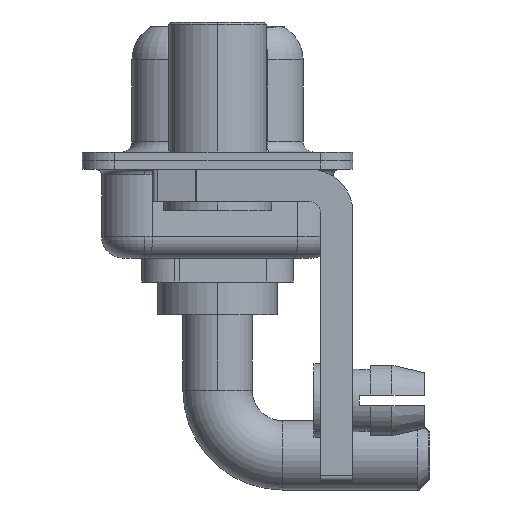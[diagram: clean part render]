
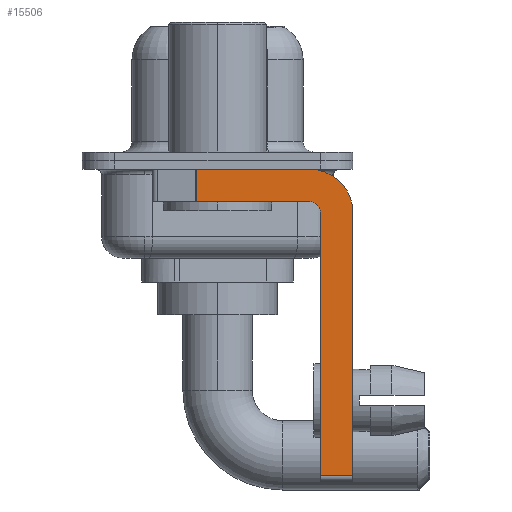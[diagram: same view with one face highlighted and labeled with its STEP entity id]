
A CAD part, left-side view. The second image highlights one B-rep face of the part: STEP entity #15506.
In plain terms, the highlighted planar face has unit normal (-1, 0, 0).
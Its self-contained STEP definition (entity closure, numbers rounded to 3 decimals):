
#155 = CARTESIAN_POINT ( 'NONE',  ( -2.9, -4.75, -2.4 ) ) ;
#188 = EDGE_CURVE ( 'NONE', #5756, #12203, #13516, .T. ) ;
#191 = PLANE ( 'NONE',  #10311 ) ;
#563 = VECTOR ( 'NONE', #5651, 1000. ) ;
#1056 = VERTEX_POINT ( 'NONE', #3633 ) ;
#1545 = ORIENTED_EDGE ( 'NONE', *, *, #10931, .F. ) ;
#1549 = CARTESIAN_POINT ( 'NONE',  ( -2.9, 0.978, -1.9 ) ) ;
#1575 = CARTESIAN_POINT ( 'NONE',  ( -2.9, -4.25, -14.55 ) ) ;
#2806 = CIRCLE ( 'NONE', #4302, 2. ) ;
#2824 = EDGE_CURVE ( 'NONE', #4322, #5120, #13715, .T. ) ;
#3224 = ORIENTED_EDGE ( 'NONE', *, *, #15464, .F. ) ;
#3633 = CARTESIAN_POINT ( 'NONE',  ( -2.9, -4.25, -0.4 ) ) ;
#4158 = DIRECTION ( 'NONE',  ( 1., 0., 0. ) ) ;
#4302 = AXIS2_PLACEMENT_3D ( 'NONE', #16575, #4158, #4515 ) ;
#4322 = VERTEX_POINT ( 'NONE', #9984 ) ;
#4487 = DIRECTION ( 'NONE',  ( -1., 0., 0. ) ) ;
#4515 = DIRECTION ( 'NONE',  ( 0., 0., -1. ) ) ;
#4554 = EDGE_CURVE ( 'NONE', #4322, #5756, #16165, .T. ) ;
#5057 = VECTOR ( 'NONE', #6839, 1000. ) ;
#5118 = CARTESIAN_POINT ( 'NONE',  ( -2.9, 3., -0.4 ) ) ;
#5120 = VERTEX_POINT ( 'NONE', #5518 ) ;
#5518 = CARTESIAN_POINT ( 'NONE',  ( -2.9, -6.25, -14.55 ) ) ;
#5614 = FACE_OUTER_BOUND ( 'NONE', #17122, .T. ) ;
#5629 = CARTESIAN_POINT ( 'NONE',  ( -2.9, -4.75, -14.8 ) ) ;
#5651 = DIRECTION ( 'NONE',  ( 0., -1., 0. ) ) ;
#5690 = AXIS2_PLACEMENT_3D ( 'NONE', #16894, #4487, #11078 ) ;
#5756 = VERTEX_POINT ( 'NONE', #155 ) ;
#5788 = ORIENTED_EDGE ( 'NONE', *, *, #4554, .F. ) ;
#5887 = LINE ( 'NONE', #1549, #11136 ) ;
#6839 = DIRECTION ( 'NONE',  ( 0., 0., -1. ) ) ;
#7161 = DIRECTION ( 'NONE',  ( 1., 0., 0. ) ) ;
#7304 = EDGE_CURVE ( 'NONE', #14701, #5120, #10545, .T. ) ;
#8168 = DIRECTION ( 'NONE',  ( 0., 0., 1. ) ) ;
#8398 = CARTESIAN_POINT ( 'NONE',  ( -2.9, -4.25, -1.9 ) ) ;
#8458 = CARTESIAN_POINT ( 'NONE',  ( -2.9, -6.25, -2.4 ) ) ;
#8648 = VERTEX_POINT ( 'NONE', #11760 ) ;
#8921 = ORIENTED_EDGE ( 'NONE', *, *, #188, .F. ) ;
#9684 = LINE ( 'NONE', #12331, #11187 ) ;
#9984 = CARTESIAN_POINT ( 'NONE',  ( -2.9, -4.75, -14.55 ) ) ;
#10311 = AXIS2_PLACEMENT_3D ( 'NONE', #12509, #7161, #17876 ) ;
#10453 = EDGE_CURVE ( 'NONE', #1056, #14701, #2806, .T. ) ;
#10545 = LINE ( 'NONE', #14737, #5057 ) ;
#10931 = EDGE_CURVE ( 'NONE', #14274, #1056, #14447, .T. ) ;
#11032 = VECTOR ( 'NONE', #8168, 1000. ) ;
#11078 = DIRECTION ( 'NONE',  ( 0., 0., 1. ) ) ;
#11105 = VECTOR ( 'NONE', #14719, 1000. ) ;
#11136 = VECTOR ( 'NONE', #16867, 1000. ) ;
#11187 = VECTOR ( 'NONE', #13967, 1000. ) ;
#11760 = CARTESIAN_POINT ( 'NONE',  ( -2.9, 0.978, -1.9 ) ) ;
#11834 = ORIENTED_EDGE ( 'NONE', *, *, #7304, .F. ) ;
#12203 = VERTEX_POINT ( 'NONE', #8398 ) ;
#12331 = CARTESIAN_POINT ( 'NONE',  ( -2.9, -4.25, -1.9 ) ) ;
#12509 = CARTESIAN_POINT ( 'NONE',  ( -2.9, -4.25, -2.4 ) ) ;
#13145 = EDGE_CURVE ( 'NONE', #14274, #8648, #5887, .T. ) ;
#13459 = CARTESIAN_POINT ( 'NONE',  ( -2.9, 0.978, -0.4 ) ) ;
#13516 = CIRCLE ( 'NONE', #5690, 0.5 ) ;
#13715 = LINE ( 'NONE', #1575, #563 ) ;
#13967 = DIRECTION ( 'NONE',  ( 0., 1., 0. ) ) ;
#14274 = VERTEX_POINT ( 'NONE', #13459 ) ;
#14447 = LINE ( 'NONE', #5118, #11105 ) ;
#14701 = VERTEX_POINT ( 'NONE', #8458 ) ;
#14719 = DIRECTION ( 'NONE',  ( 0., -1., 0. ) ) ;
#14737 = CARTESIAN_POINT ( 'NONE',  ( -2.9, -6.25, -2.4 ) ) ;
#15464 = EDGE_CURVE ( 'NONE', #12203, #8648, #9684, .T. ) ;
#15506 = ADVANCED_FACE ( 'NONE', ( #5614 ), #191, .F. ) ;
#16165 = LINE ( 'NONE', #5629, #11032 ) ;
#16416 = ORIENTED_EDGE ( 'NONE', *, *, #13145, .T. ) ;
#16575 = CARTESIAN_POINT ( 'NONE',  ( -2.9, -4.25, -2.4 ) ) ;
#16867 = DIRECTION ( 'NONE',  ( 0., 0., -1. ) ) ;
#16894 = CARTESIAN_POINT ( 'NONE',  ( -2.9, -4.25, -2.4 ) ) ;
#17122 = EDGE_LOOP ( 'NONE', ( #1545, #16416, #3224, #8921, #5788, #17784, #11834, #17774 ) ) ;
#17774 = ORIENTED_EDGE ( 'NONE', *, *, #10453, .F. ) ;
#17784 = ORIENTED_EDGE ( 'NONE', *, *, #2824, .T. ) ;
#17876 = DIRECTION ( 'NONE',  ( 0., 0., -1. ) ) ;
